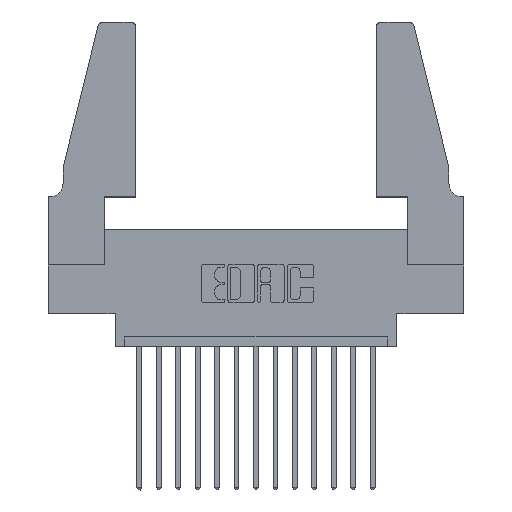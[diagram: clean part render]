
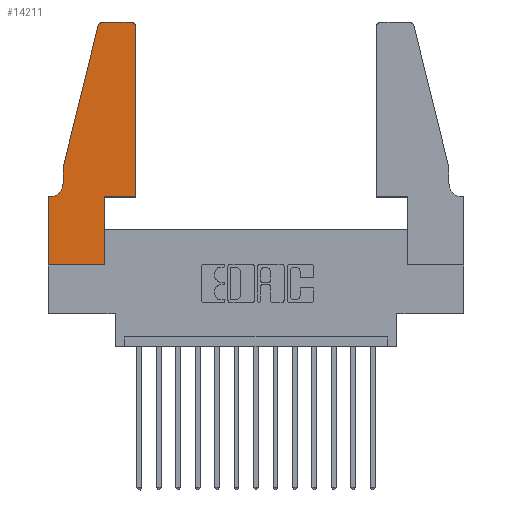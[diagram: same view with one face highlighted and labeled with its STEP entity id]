
A CAD part, top view. The second image highlights one B-rep face of the part: STEP entity #14211.
In plain terms, the highlighted planar face has unit normal (0, 0, 1).
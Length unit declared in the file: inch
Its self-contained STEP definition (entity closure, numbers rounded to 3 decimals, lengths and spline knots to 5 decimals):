
#58 = VERTEX_POINT ( 'NONE', #9213 ) ;
#169 = ORIENTED_EDGE ( 'NONE', *, *, #5421, .T. ) ;
#614 = EDGE_CURVE ( 'NONE', #8453, #15629, #3520, .T. ) ;
#680 = DIRECTION ( 'NONE',  ( -1., 0., 0. ) ) ;
#790 = ORIENTED_EDGE ( 'NONE', *, *, #6189, .T. ) ;
#794 = VECTOR ( 'NONE', #5785, 39.37008 ) ;
#1657 = DIRECTION ( 'NONE',  ( 0., 1., 0. ) ) ;
#1760 = AXIS2_PLACEMENT_3D ( 'NONE', #12062, #14411, #14579 ) ;
#1867 = LINE ( 'NONE', #12020, #6167 ) ;
#1959 = EDGE_CURVE ( 'NONE', #5283, #2784, #1867, .T. ) ;
#1994 = VERTEX_POINT ( 'NONE', #10753 ) ;
#2147 = VERTEX_POINT ( 'NONE', #8528 ) ;
#2585 = VECTOR ( 'NONE', #6872, 39.37008 ) ;
#2595 = ORIENTED_EDGE ( 'NONE', *, *, #13215, .T. ) ;
#2729 = CARTESIAN_POINT ( 'NONE',  ( 0.2865, 0.35, 0.37 ) ) ;
#2784 = VERTEX_POINT ( 'NONE', #12279 ) ;
#2943 = LINE ( 'NONE', #11157, #4682 ) ;
#3094 = LINE ( 'NONE', #15707, #8318 ) ;
#3204 = DIRECTION ( 'NONE',  ( 1., 0., 0. ) ) ;
#3431 = DIRECTION ( 'NONE',  ( 1., 0., 0. ) ) ;
#3449 = ORIENTED_EDGE ( 'NONE', *, *, #4150, .T. ) ;
#3508 = ORIENTED_EDGE ( 'NONE', *, *, #3559, .T. ) ;
#3520 = LINE ( 'NONE', #2729, #6999 ) ;
#3559 = EDGE_CURVE ( 'NONE', #1994, #5283, #15341, .T. ) ;
#3811 = LINE ( 'NONE', #12545, #6513 ) ;
#4150 = EDGE_CURVE ( 'NONE', #14817, #2147, #9573, .T. ) ;
#4682 = VECTOR ( 'NONE', #13574, 39.37008 ) ;
#4893 = EDGE_CURVE ( 'NONE', #58, #14817, #7205, .T. ) ;
#5194 = DIRECTION ( 'NONE',  ( 0., 1., 0. ) ) ;
#5283 = VERTEX_POINT ( 'NONE', #11898 ) ;
#5421 = EDGE_CURVE ( 'NONE', #2784, #58, #2943, .T. ) ;
#5609 = AXIS2_PLACEMENT_3D ( 'NONE', #12917, #11923, #3204 ) ;
#5748 = CARTESIAN_POINT ( 'NONE',  ( 0., 0., 0.37 ) ) ;
#5783 = EDGE_CURVE ( 'NONE', #15629, #13243, #14662, .T. ) ;
#5785 = DIRECTION ( 'NONE',  ( 1., 0., 0. ) ) ;
#5970 = FACE_OUTER_BOUND ( 'NONE', #9473, .T. ) ;
#6167 = VECTOR ( 'NONE', #15595, 39.37008 ) ;
#6189 = EDGE_CURVE ( 'NONE', #2147, #6295, #3094, .T. ) ;
#6295 = VERTEX_POINT ( 'NONE', #13802 ) ;
#6513 = VECTOR ( 'NONE', #1657, 39.37008 ) ;
#6642 = ORIENTED_EDGE ( 'NONE', *, *, #1959, .T. ) ;
#6678 = EDGE_CURVE ( 'NONE', #13856, #1994, #14037, .T. ) ;
#6710 = CIRCLE ( 'NONE', #7207, 0.03 ) ;
#6872 = DIRECTION ( 'NONE',  ( -1., 0., 0. ) ) ;
#6991 = DIRECTION ( 'NONE',  ( 0., -1., 0. ) ) ;
#6992 = PLANE ( 'NONE',  #5609 ) ;
#6999 = VECTOR ( 'NONE', #5194, 39.37008 ) ;
#7205 = CIRCLE ( 'NONE', #1760, 0.07 ) ;
#7207 = AXIS2_PLACEMENT_3D ( 'NONE', #8781, #9949, #9897 ) ;
#7878 = CARTESIAN_POINT ( 'NONE',  ( 0.0755, 0.35, 0.37 ) ) ;
#8177 = ORIENTED_EDGE ( 'NONE', *, *, #14651, .T. ) ;
#8318 = VECTOR ( 'NONE', #6991, 39.37008 ) ;
#8453 = VERTEX_POINT ( 'NONE', #13235 ) ;
#8528 = CARTESIAN_POINT ( 'NONE',  ( 0., 0.35, 0.37 ) ) ;
#8781 = CARTESIAN_POINT ( 'NONE',  ( 0.4205, 1.22, 0.37 ) ) ;
#8820 = VERTEX_POINT ( 'NONE', #10198 ) ;
#8898 = CARTESIAN_POINT ( 'NONE',  ( 0.2605, 1.25, 0.37 ) ) ;
#8990 = ORIENTED_EDGE ( 'NONE', *, *, #4893, .T. ) ;
#9119 = EDGE_CURVE ( 'NONE', #8820, #13856, #6710, .T. ) ;
#9213 = CARTESIAN_POINT ( 'NONE',  ( 0.0755, 0.42, 0.37 ) ) ;
#9473 = EDGE_LOOP ( 'NONE', ( #10600, #3508, #6642, #169, #8990, #3449, #790, #2595, #12173, #10081, #8177, #14224 ) ) ;
#9573 = LINE ( 'NONE', #7878, #2585 ) ;
#9897 = DIRECTION ( 'NONE',  ( 1., 0., 0. ) ) ;
#9949 = DIRECTION ( 'NONE',  ( 0., 0., 1. ) ) ;
#9978 = AXIS2_PLACEMENT_3D ( 'NONE', #11463, #11564, #12874 ) ;
#10081 = ORIENTED_EDGE ( 'NONE', *, *, #5783, .T. ) ;
#10198 = CARTESIAN_POINT ( 'NONE',  ( 0.4505, 1.22, 0.37 ) ) ;
#10244 = VECTOR ( 'NONE', #3431, 39.37008 ) ;
#10600 = ORIENTED_EDGE ( 'NONE', *, *, #6678, .T. ) ;
#10700 = CARTESIAN_POINT ( 'NONE',  ( 0.4505, 0.35, 0.37 ) ) ;
#10753 = CARTESIAN_POINT ( 'NONE',  ( 0.284, 1.25, 0.37 ) ) ;
#10890 = CARTESIAN_POINT ( 'NONE',  ( 0.2865, 0.35, 0.37 ) ) ;
#11157 = CARTESIAN_POINT ( 'NONE',  ( 0.0755, 0.5, 0.37 ) ) ;
#11463 = CARTESIAN_POINT ( 'NONE',  ( 0.284, 1.22, 0.37 ) ) ;
#11564 = DIRECTION ( 'NONE',  ( 0., 0., 1. ) ) ;
#11588 = CARTESIAN_POINT ( 'NONE',  ( 0.0055, 0.35, 0.37 ) ) ;
#11898 = CARTESIAN_POINT ( 'NONE',  ( 0.25487, 1.22718, 0.37 ) ) ;
#11923 = DIRECTION ( 'NONE',  ( 0., 0., 1. ) ) ;
#12020 = CARTESIAN_POINT ( 'NONE',  ( 0.0755, 0.5, 0.37 ) ) ;
#12062 = CARTESIAN_POINT ( 'NONE',  ( 0.0055, 0.42, 0.37 ) ) ;
#12173 = ORIENTED_EDGE ( 'NONE', *, *, #614, .T. ) ;
#12279 = CARTESIAN_POINT ( 'NONE',  ( 0.0755, 0.5, 0.37 ) ) ;
#12545 = CARTESIAN_POINT ( 'NONE',  ( 0.4505, 0.35, 0.37 ) ) ;
#12874 = DIRECTION ( 'NONE',  ( 1., 0., 0. ) ) ;
#12917 = CARTESIAN_POINT ( 'NONE',  ( 0., 0.35, 0.37 ) ) ;
#13215 = EDGE_CURVE ( 'NONE', #6295, #8453, #14821, .T. ) ;
#13235 = CARTESIAN_POINT ( 'NONE',  ( 0.2865, 0., 0.37 ) ) ;
#13243 = VERTEX_POINT ( 'NONE', #14458 ) ;
#13574 = DIRECTION ( 'NONE',  ( 0., -1., 0. ) ) ;
#13641 = VECTOR ( 'NONE', #680, 39.37008 ) ;
#13802 = CARTESIAN_POINT ( 'NONE',  ( 0., 0., 0.37 ) ) ;
#13856 = VERTEX_POINT ( 'NONE', #15660 ) ;
#14037 = LINE ( 'NONE', #8898, #13641 ) ;
#14211 = ADVANCED_FACE ( 'NONE', ( #5970 ), #6992, .T. ) ;
#14224 = ORIENTED_EDGE ( 'NONE', *, *, #9119, .T. ) ;
#14411 = DIRECTION ( 'NONE',  ( 0., 0., -1. ) ) ;
#14458 = CARTESIAN_POINT ( 'NONE',  ( 0.4505, 0.35, 0.37 ) ) ;
#14579 = DIRECTION ( 'NONE',  ( -1., 0., 0. ) ) ;
#14651 = EDGE_CURVE ( 'NONE', #13243, #8820, #3811, .T. ) ;
#14662 = LINE ( 'NONE', #10700, #794 ) ;
#14817 = VERTEX_POINT ( 'NONE', #11588 ) ;
#14821 = LINE ( 'NONE', #5748, #10244 ) ;
#15341 = CIRCLE ( 'NONE', #9978, 0.03 ) ;
#15595 = DIRECTION ( 'NONE',  ( -0.239, -0.971, 0. ) ) ;
#15629 = VERTEX_POINT ( 'NONE', #10890 ) ;
#15660 = CARTESIAN_POINT ( 'NONE',  ( 0.4205, 1.25, 0.37 ) ) ;
#15707 = CARTESIAN_POINT ( 'NONE',  ( 0., 0., 0.37 ) ) ;
